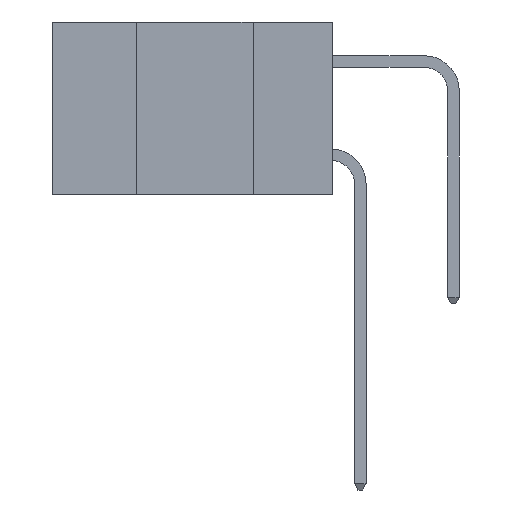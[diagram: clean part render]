
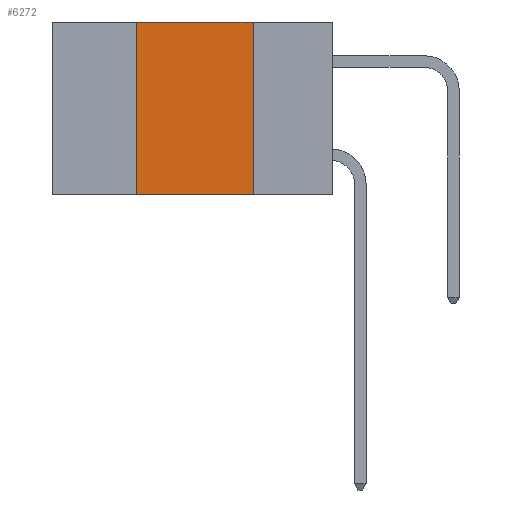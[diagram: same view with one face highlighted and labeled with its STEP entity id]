
A CAD part, left-side view. The second image highlights one B-rep face of the part: STEP entity #6272.
In plain terms, the highlighted planar face has unit normal (-1, 0, 0).
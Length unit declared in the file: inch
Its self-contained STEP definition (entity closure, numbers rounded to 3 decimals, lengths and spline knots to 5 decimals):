
#480 = LINE ( 'NONE', #10083, #27828 ) ;
#677 = EDGE_CURVE ( 'NONE', #7183, #25715, #25803, .T. ) ;
#1147 = ORIENTED_EDGE ( 'NONE', *, *, #3067, .F. ) ;
#2105 = DIRECTION ( 'NONE',  ( 0., 0., -1. ) ) ;
#3067 = EDGE_CURVE ( 'NONE', #8794, #25715, #3994, .T. ) ;
#3994 = LINE ( 'NONE', #16267, #20617 ) ;
#4938 = DIRECTION ( 'NONE',  ( 0., 0., 1. ) ) ;
#5697 = VERTEX_POINT ( 'NONE', #6794 ) ;
#6272 = ADVANCED_FACE ( 'NONE', ( #13429 ), #13007, .F. ) ;
#6307 = CARTESIAN_POINT ( 'NONE',  ( 0., 0.6, -0.37 ) ) ;
#6794 = CARTESIAN_POINT ( 'NONE',  ( 0., 0.42, 0. ) ) ;
#6833 = EDGE_CURVE ( 'NONE', #7183, #5697, #15801, .T. ) ;
#7183 = VERTEX_POINT ( 'NONE', #14620 ) ;
#7653 = ORIENTED_EDGE ( 'NONE', *, *, #6833, .F. ) ;
#8794 = VERTEX_POINT ( 'NONE', #13398 ) ;
#10083 = CARTESIAN_POINT ( 'NONE',  ( 0., 0.6, 0. ) ) ;
#12789 = ORIENTED_EDGE ( 'NONE', *, *, #23267, .F. ) ;
#13007 = PLANE ( 'NONE',  #21425 ) ;
#13256 = EDGE_LOOP ( 'NONE', ( #1147, #12789, #7653, #13464 ) ) ;
#13398 = CARTESIAN_POINT ( 'NONE',  ( 0., 0.17, 0. ) ) ;
#13429 = FACE_OUTER_BOUND ( 'NONE', #13256, .T. ) ;
#13464 = ORIENTED_EDGE ( 'NONE', *, *, #677, .T. ) ;
#13783 = CARTESIAN_POINT ( 'NONE',  ( 0., 0.17, -0.37 ) ) ;
#14620 = CARTESIAN_POINT ( 'NONE',  ( 0., 0.42, -0.37 ) ) ;
#15209 = DIRECTION ( 'NONE',  ( 1., 0., 0. ) ) ;
#15801 = LINE ( 'NONE', #18017, #17162 ) ;
#15871 = DIRECTION ( 'NONE',  ( 0., 0., -1. ) ) ;
#16267 = CARTESIAN_POINT ( 'NONE',  ( 0., 0.17, -0.37 ) ) ;
#17162 = VECTOR ( 'NONE', #4938, 39.37008 ) ;
#18017 = CARTESIAN_POINT ( 'NONE',  ( 0., 0.42, -0.37 ) ) ;
#20617 = VECTOR ( 'NONE', #15871, 39.37008 ) ;
#20766 = DIRECTION ( 'NONE',  ( 0., -1., 0. ) ) ;
#20780 = VECTOR ( 'NONE', #21939, 39.37008 ) ;
#21425 = AXIS2_PLACEMENT_3D ( 'NONE', #25789, #15209, #2105 ) ;
#21939 = DIRECTION ( 'NONE',  ( 0., -1., 0. ) ) ;
#23267 = EDGE_CURVE ( 'NONE', #5697, #8794, #480, .T. ) ;
#25715 = VERTEX_POINT ( 'NONE', #13783 ) ;
#25789 = CARTESIAN_POINT ( 'NONE',  ( 0., 0.6, 0. ) ) ;
#25803 = LINE ( 'NONE', #6307, #20780 ) ;
#27828 = VECTOR ( 'NONE', #20766, 39.37008 ) ;
